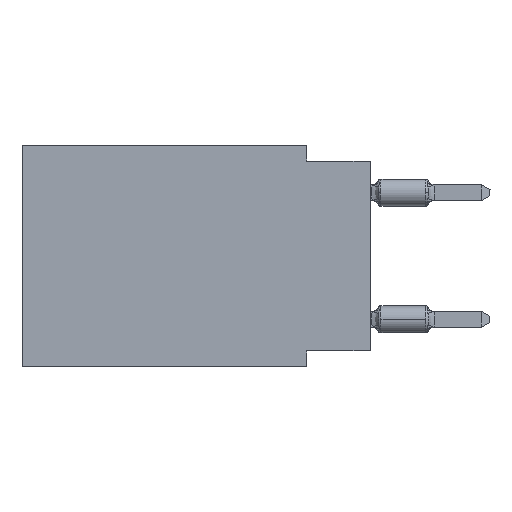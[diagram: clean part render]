
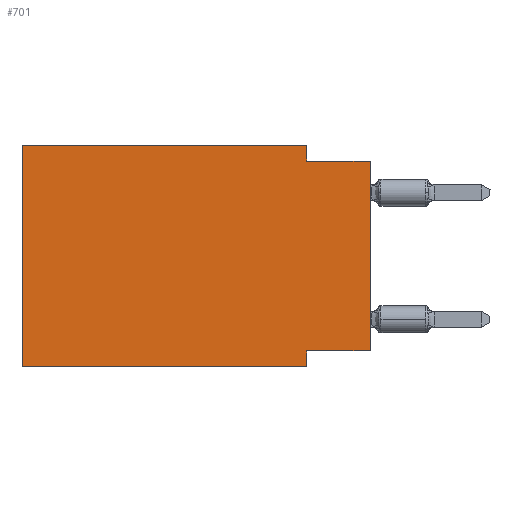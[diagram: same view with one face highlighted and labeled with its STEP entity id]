
A CAD part, left-side view. The second image highlights one B-rep face of the part: STEP entity #701.
In plain terms, the highlighted planar face has unit normal (-1, 0, 0).
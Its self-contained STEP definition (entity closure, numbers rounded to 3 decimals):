
#701 = ADVANCED_FACE ( 'NONE', ( #11228 ), #56220, .F. ) ;
#1907 = ORIENTED_EDGE ( 'NONE', *, *, #37844, .F. ) ;
#2389 = ORIENTED_EDGE ( 'NONE', *, *, #8167, .T. ) ;
#3776 = CARTESIAN_POINT ( 'NONE',  ( 0., 0., -0.635 ) ) ;
#3878 = VERTEX_POINT ( 'NONE', #42763 ) ;
#4263 = VECTOR ( 'NONE', #10037, 1000. ) ;
#4428 = VERTEX_POINT ( 'NONE', #20347 ) ;
#6812 = DIRECTION ( 'NONE',  ( 1., 0., 0. ) ) ;
#7274 = ORIENTED_EDGE ( 'NONE', *, *, #51548, .F. ) ;
#8167 = EDGE_CURVE ( 'NONE', #52632, #28031, #24745, .T. ) ;
#8511 = DIRECTION ( 'NONE',  ( 0., -1., 0. ) ) ;
#9017 = VECTOR ( 'NONE', #8511, 1000. ) ;
#9373 = CARTESIAN_POINT ( 'NONE',  ( 0., 0., -8.255 ) ) ;
#9667 = DIRECTION ( 'NONE',  ( 0., 1., 0. ) ) ;
#9752 = CARTESIAN_POINT ( 'NONE',  ( 0., 2.54, -8.89 ) ) ;
#10037 = DIRECTION ( 'NONE',  ( 0., 0., -1. ) ) ;
#11209 = CARTESIAN_POINT ( 'NONE',  ( 0., 0., 0. ) ) ;
#11228 = FACE_OUTER_BOUND ( 'NONE', #46700, .T. ) ;
#11475 = VECTOR ( 'NONE', #9667, 1000. ) ;
#13662 = EDGE_CURVE ( 'NONE', #52632, #48977, #45567, .T. ) ;
#14438 = CARTESIAN_POINT ( 'NONE',  ( 0., 13.97, -8.89 ) ) ;
#20347 = CARTESIAN_POINT ( 'NONE',  ( 0., 13.97, -8.89 ) ) ;
#21148 = VECTOR ( 'NONE', #32506, 1000. ) ;
#22002 = LINE ( 'NONE', #3776, #49278 ) ;
#22245 = VERTEX_POINT ( 'NONE', #31088 ) ;
#24745 = LINE ( 'NONE', #11209, #29432 ) ;
#28031 = VERTEX_POINT ( 'NONE', #40832 ) ;
#28382 = CARTESIAN_POINT ( 'NONE',  ( 0., 2.54, -8.255 ) ) ;
#29160 = DIRECTION ( 'NONE',  ( 0., 0., 1. ) ) ;
#29432 = VECTOR ( 'NONE', #29160, 1000. ) ;
#31088 = CARTESIAN_POINT ( 'NONE',  ( 0., 2.54, -8.89 ) ) ;
#32506 = DIRECTION ( 'NONE',  ( 0., 0., -1. ) ) ;
#32678 = LINE ( 'NONE', #9752, #4263 ) ;
#33179 = CARTESIAN_POINT ( 'NONE',  ( 0., 0., -8.255 ) ) ;
#33545 = LINE ( 'NONE', #47382, #9017 ) ;
#34461 = CARTESIAN_POINT ( 'NONE',  ( 0., 13.97, 0. ) ) ;
#36308 = AXIS2_PLACEMENT_3D ( 'NONE', #34461, #6812, #52393 ) ;
#36563 = CARTESIAN_POINT ( 'NONE',  ( 0., 2.54, -0.635 ) ) ;
#36721 = ORIENTED_EDGE ( 'NONE', *, *, #43849, .F. ) ;
#37122 = ORIENTED_EDGE ( 'NONE', *, *, #52213, .F. ) ;
#37844 = EDGE_CURVE ( 'NONE', #4428, #3878, #43088, .T. ) ;
#38781 = DIRECTION ( 'NONE',  ( 0., -1., 0. ) ) ;
#38970 = CARTESIAN_POINT ( 'NONE',  ( 0., 13.97, 0. ) ) ;
#39493 = VERTEX_POINT ( 'NONE', #36563 ) ;
#39996 = ORIENTED_EDGE ( 'NONE', *, *, #44297, .F. ) ;
#40804 = VERTEX_POINT ( 'NONE', #47157 ) ;
#40832 = CARTESIAN_POINT ( 'NONE',  ( 0., 0., -0.635 ) ) ;
#41622 = LINE ( 'NONE', #53998, #21148 ) ;
#42763 = CARTESIAN_POINT ( 'NONE',  ( 0., 13.97, 0. ) ) ;
#43088 = LINE ( 'NONE', #38970, #55394 ) ;
#43305 = ORIENTED_EDGE ( 'NONE', *, *, #51976, .T. ) ;
#43849 = EDGE_CURVE ( 'NONE', #39493, #28031, #22002, .T. ) ;
#44297 = EDGE_CURVE ( 'NONE', #48977, #22245, #32678, .T. ) ;
#45567 = LINE ( 'NONE', #9373, #11475 ) ;
#45908 = LINE ( 'NONE', #14438, #56903 ) ;
#46700 = EDGE_LOOP ( 'NONE', ( #2389, #36721, #7274, #37122, #1907, #43305, #39996, #53220 ) ) ;
#47157 = CARTESIAN_POINT ( 'NONE',  ( 0., 2.54, 0. ) ) ;
#47382 = CARTESIAN_POINT ( 'NONE',  ( 0., 13.97, 0. ) ) ;
#48977 = VERTEX_POINT ( 'NONE', #28382 ) ;
#49278 = VECTOR ( 'NONE', #38781, 1000. ) ;
#50915 = DIRECTION ( 'NONE',  ( 0., -1., 0. ) ) ;
#51548 = EDGE_CURVE ( 'NONE', #40804, #39493, #41622, .T. ) ;
#51624 = DIRECTION ( 'NONE',  ( 0., 0., 1. ) ) ;
#51976 = EDGE_CURVE ( 'NONE', #4428, #22245, #45908, .T. ) ;
#52213 = EDGE_CURVE ( 'NONE', #3878, #40804, #33545, .T. ) ;
#52393 = DIRECTION ( 'NONE',  ( 0., 0., -1. ) ) ;
#52632 = VERTEX_POINT ( 'NONE', #33179 ) ;
#53220 = ORIENTED_EDGE ( 'NONE', *, *, #13662, .F. ) ;
#53998 = CARTESIAN_POINT ( 'NONE',  ( 0., 2.54, 0. ) ) ;
#55394 = VECTOR ( 'NONE', #51624, 1000. ) ;
#56220 = PLANE ( 'NONE',  #36308 ) ;
#56903 = VECTOR ( 'NONE', #50915, 1000. ) ;
